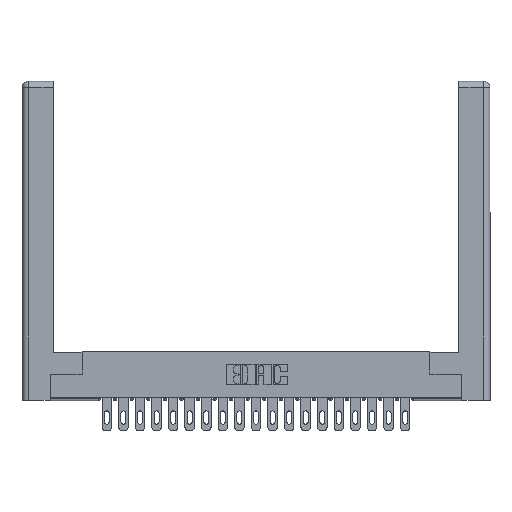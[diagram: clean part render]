
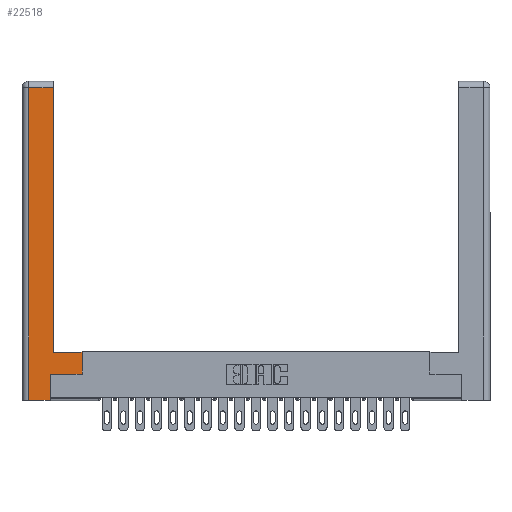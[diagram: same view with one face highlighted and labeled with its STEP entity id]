
A CAD part, top view. The second image highlights one B-rep face of the part: STEP entity #22518.
In plain terms, the highlighted planar face has unit normal (0, 0, 1).
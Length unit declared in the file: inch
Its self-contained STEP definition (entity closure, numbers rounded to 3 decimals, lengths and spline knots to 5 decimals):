
#1154 = LINE ( 'NONE', #19595, #6262 ) ;
#1258 = LINE ( 'NONE', #15153, #17942 ) ;
#1801 = ORIENTED_EDGE ( 'NONE', *, *, #4360, .T. ) ;
#2238 = VERTEX_POINT ( 'NONE', #22044 ) ;
#2419 = CARTESIAN_POINT ( 'NONE',  ( 0.265, 0., 0. ) ) ;
#2618 = VERTEX_POINT ( 'NONE', #9329 ) ;
#2784 = DIRECTION ( 'NONE',  ( 0., -1., 0. ) ) ;
#2816 = CARTESIAN_POINT ( 'NONE',  ( 0.565, 0.245, 0. ) ) ;
#2858 = LINE ( 'NONE', #2816, #6675 ) ;
#2955 = ORIENTED_EDGE ( 'NONE', *, *, #15036, .T. ) ;
#3174 = VERTEX_POINT ( 'NONE', #2419 ) ;
#3338 = CARTESIAN_POINT ( 'NONE',  ( 0.295, 0.45, 0. ) ) ;
#3596 = ORIENTED_EDGE ( 'NONE', *, *, #3622, .T. ) ;
#3622 = EDGE_CURVE ( 'NONE', #13702, #18914, #1154, .T. ) ;
#4360 = EDGE_CURVE ( 'NONE', #13744, #14968, #16580, .T. ) ;
#4390 = DIRECTION ( 'NONE',  ( 0., 1., 0. ) ) ;
#4806 = DIRECTION ( 'NONE',  ( -1., 0., 0. ) ) ;
#4891 = EDGE_CURVE ( 'NONE', #14968, #3174, #17487, .T. ) ;
#5143 = CARTESIAN_POINT ( 'NONE',  ( 0., 0., 0. ) ) ;
#5439 = LINE ( 'NONE', #16435, #24891 ) ;
#5457 = CARTESIAN_POINT ( 'NONE',  ( 0.265, 0., 0. ) ) ;
#6262 = VECTOR ( 'NONE', #15943, 39.37008 ) ;
#6675 = VECTOR ( 'NONE', #18788, 39.37008 ) ;
#6846 = VECTOR ( 'NONE', #2784, 39.37008 ) ;
#7402 = ORIENTED_EDGE ( 'NONE', *, *, #8830, .T. ) ;
#8127 = CARTESIAN_POINT ( 'NONE',  ( 0.0615, 2.94, 0. ) ) ;
#8455 = CARTESIAN_POINT ( 'NONE',  ( 0.0615, 0., 0. ) ) ;
#8759 = EDGE_CURVE ( 'NONE', #17027, #2238, #2858, .T. ) ;
#8830 = EDGE_CURVE ( 'NONE', #2618, #13702, #17010, .T. ) ;
#9067 = DIRECTION ( 'NONE',  ( 0., 0., -1. ) ) ;
#9329 = CARTESIAN_POINT ( 'NONE',  ( 0.565, 0.45, 0. ) ) ;
#10620 = ORIENTED_EDGE ( 'NONE', *, *, #15177, .T. ) ;
#10705 = DIRECTION ( 'NONE',  ( -1., 0., 0. ) ) ;
#13252 = CARTESIAN_POINT ( 'NONE',  ( 0.0615, 0., 0. ) ) ;
#13647 = EDGE_LOOP ( 'NONE', ( #3596, #2955, #1801, #18792, #10620, #16162, #14155, #7402 ) ) ;
#13702 = VERTEX_POINT ( 'NONE', #21614 ) ;
#13744 = VERTEX_POINT ( 'NONE', #8127 ) ;
#13877 = EDGE_CURVE ( 'NONE', #2238, #2618, #5439, .T. ) ;
#14155 = ORIENTED_EDGE ( 'NONE', *, *, #13877, .T. ) ;
#14830 = PLANE ( 'NONE',  #24868 ) ;
#14837 = LINE ( 'NONE', #16669, #17024 ) ;
#14968 = VERTEX_POINT ( 'NONE', #8455 ) ;
#15036 = EDGE_CURVE ( 'NONE', #18914, #13744, #14837, .T. ) ;
#15153 = CARTESIAN_POINT ( 'NONE',  ( 0.265, 0.245, 0. ) ) ;
#15177 = EDGE_CURVE ( 'NONE', #3174, #17027, #1258, .T. ) ;
#15388 = FACE_OUTER_BOUND ( 'NONE', #13647, .T. ) ;
#15594 = DIRECTION ( 'NONE',  ( 1., 0., 0. ) ) ;
#15943 = DIRECTION ( 'NONE',  ( 0., 1., 0. ) ) ;
#16162 = ORIENTED_EDGE ( 'NONE', *, *, #8759, .T. ) ;
#16435 = CARTESIAN_POINT ( 'NONE',  ( 0.565, 0.45, 0. ) ) ;
#16580 = LINE ( 'NONE', #13252, #6846 ) ;
#16669 = CARTESIAN_POINT ( 'NONE',  ( 0.0615, 2.94, 0. ) ) ;
#17010 = LINE ( 'NONE', #3338, #22350 ) ;
#17024 = VECTOR ( 'NONE', #10705, 39.37008 ) ;
#17027 = VERTEX_POINT ( 'NONE', #25034 ) ;
#17487 = LINE ( 'NONE', #5457, #19012 ) ;
#17942 = VECTOR ( 'NONE', #23290, 39.37008 ) ;
#18788 = DIRECTION ( 'NONE',  ( 1., 0., 0. ) ) ;
#18792 = ORIENTED_EDGE ( 'NONE', *, *, #4891, .T. ) ;
#18914 = VERTEX_POINT ( 'NONE', #20849 ) ;
#19012 = VECTOR ( 'NONE', #15594, 39.37008 ) ;
#19595 = CARTESIAN_POINT ( 'NONE',  ( 0.295, 3., 0. ) ) ;
#20849 = CARTESIAN_POINT ( 'NONE',  ( 0.295, 2.94, 0. ) ) ;
#21614 = CARTESIAN_POINT ( 'NONE',  ( 0.295, 0.45, 0. ) ) ;
#22044 = CARTESIAN_POINT ( 'NONE',  ( 0.565, 0.245, 0. ) ) ;
#22350 = VECTOR ( 'NONE', #23428, 39.37008 ) ;
#22518 = ADVANCED_FACE ( 'NONE', ( #15388 ), #14830, .F. ) ;
#23290 = DIRECTION ( 'NONE',  ( 0., 1., 0. ) ) ;
#23428 = DIRECTION ( 'NONE',  ( -1., 0., 0. ) ) ;
#24868 = AXIS2_PLACEMENT_3D ( 'NONE', #5143, #9067, #4806 ) ;
#24891 = VECTOR ( 'NONE', #4390, 39.37008 ) ;
#25034 = CARTESIAN_POINT ( 'NONE',  ( 0.265, 0.245, 0. ) ) ;
